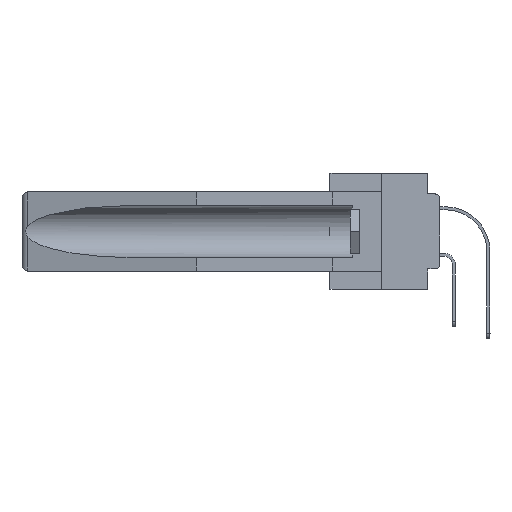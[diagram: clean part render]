
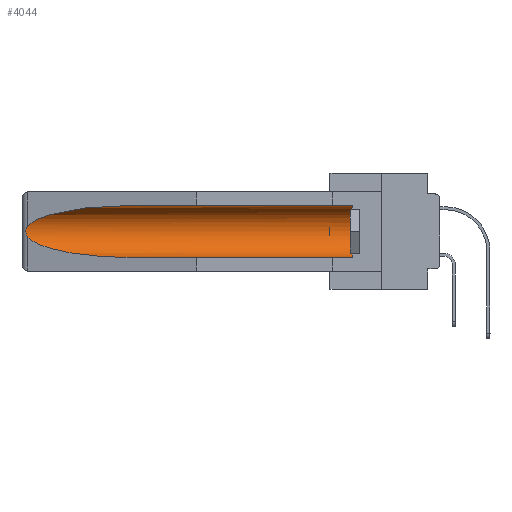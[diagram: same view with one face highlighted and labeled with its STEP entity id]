
A CAD part, left-side view. The second image highlights one B-rep face of the part: STEP entity #4044.
In plain terms, the highlighted cylindrical face has radius 2.857 mm (diameter 5.715 mm), a partial arc.
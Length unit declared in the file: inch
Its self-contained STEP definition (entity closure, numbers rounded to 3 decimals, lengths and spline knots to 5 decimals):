
#299 = CIRCLE ( 'NONE', #5809, 0.1125 ) ;
#533 = ORIENTED_EDGE ( 'NONE', *, *, #35859, .T. ) ;
#1902 = ORIENTED_EDGE ( 'NONE', *, *, #36746, .T. ) ;
#4044 = ADVANCED_FACE ( 'NONE', ( #23453 ), #39282, .F. ) ;
#4335 = CARTESIAN_POINT ( 'NONE',  ( 0.21114, 1.30732, -0.059 ) ) ;
#4344 = DIRECTION ( 'NONE',  ( 0., 1., 0. ) ) ;
#4730 = ORIENTED_EDGE ( 'NONE', *, *, #24050, .F. ) ;
#5407 = ORIENTED_EDGE ( 'NONE', *, *, #29648, .T. ) ;
#5632 = VERTEX_POINT ( 'NONE', #34740 ) ;
#5809 = AXIS2_PLACEMENT_3D ( 'NONE', #38741, #35045, #41558 ) ;
#7453 = CARTESIAN_POINT ( 'NONE',  ( 0.2675, 1.53308, -0.16763 ) ) ;
#7535 =( BOUNDED_CURVE ( )  B_SPLINE_CURVE ( 3, ( #8912, #19321, #12401, #36028 ),
 .UNSPECIFIED., .F., .F. ) 
 B_SPLINE_CURVE_WITH_KNOTS ( ( 4, 4 ),
 ( 0.1948, 1.5708 ),
 .UNSPECIFIED. ) 
 CURVE ( )  GEOMETRIC_REPRESENTATION_ITEM ( )  RATIONAL_B_SPLINE_CURVE ( ( 1., 0.848, 0.848, 1. ) ) 
 REPRESENTATION_ITEM ( '' )  );
#8299 = VECTOR ( 'NONE', #28967, 39.37008 ) ;
#8912 = CARTESIAN_POINT ( 'NONE',  ( 0.26537, 1.52718, -0.19328 ) ) ;
#8949 = CARTESIAN_POINT ( 'NONE',  ( 0.155, 1.07973, -0.284 ) ) ;
#11121 = CARTESIAN_POINT ( 'NONE',  ( 0.26597, 1.5296, -0.19026 ) ) ;
#12401 = CARTESIAN_POINT ( 'NONE',  ( 0.21114, 1.30732, -0.284 ) ) ;
#14147 = CARTESIAN_POINT ( 'NONE',  ( 0.2673, 1.5327, -0.16383 ) ) ;
#15965 = LINE ( 'NONE', #32635, #8299 ) ;
#16817 = CARTESIAN_POINT ( 'NONE',  ( 0.155, 0.126, -0.059 ) ) ;
#16933 = VERTEX_POINT ( 'NONE', #17651 ) ;
#17651 = CARTESIAN_POINT ( 'NONE',  ( 0.155, 1.07973, -0.059 ) ) ;
#17791 = AXIS2_PLACEMENT_3D ( 'NONE', #19331, #32550, #42531 ) ;
#18020 = CARTESIAN_POINT ( 'NONE',  ( 0.155, 0.126, -0.284 ) ) ;
#18270 =( BOUNDED_CURVE ( )  B_SPLINE_CURVE ( 3, ( #20996, #4335, #34221, #30986 ),
 .UNSPECIFIED., .F., .F. ) 
 B_SPLINE_CURVE_WITH_KNOTS ( ( 4, 4 ),
 ( 4.71239, 6.08839 ),
 .UNSPECIFIED. ) 
 CURVE ( )  GEOMETRIC_REPRESENTATION_ITEM ( )  RATIONAL_B_SPLINE_CURVE ( ( 1., 0.848, 0.848, 1. ) ) 
 REPRESENTATION_ITEM ( '' )  );
#19048 = EDGE_CURVE ( 'NONE', #34574, #16933, #34019, .T. ) ;
#19321 = CARTESIAN_POINT ( 'NONE',  ( 0.25451, 1.48313, -0.24835 ) ) ;
#19331 = CARTESIAN_POINT ( 'NONE',  ( 0.155, -0.30754, -0.1715 ) ) ;
#20863 = CARTESIAN_POINT ( 'NONE',  ( 0.2675, 1.53308, -0.17534 ) ) ;
#20996 = CARTESIAN_POINT ( 'NONE',  ( 0.155, 1.07973, -0.059 ) ) ;
#23453 = FACE_OUTER_BOUND ( 'NONE', #29745, .T. ) ;
#24050 = EDGE_CURVE ( 'NONE', #32086, #33594, #15965, .T. ) ;
#27362 = VECTOR ( 'NONE', #4344, 39.37008 ) ;
#27600 = CARTESIAN_POINT ( 'NONE',  ( 0.26655, 1.53094, -0.18657 ) ) ;
#28967 = DIRECTION ( 'NONE',  ( 0., 1., 0. ) ) ;
#29648 = EDGE_CURVE ( 'NONE', #16933, #35137, #18270, .T. ) ;
#29745 = EDGE_LOOP ( 'NONE', ( #5407, #38302, #533, #4730, #1902, #31126 ) ) ;
#30202 = CARTESIAN_POINT ( 'NONE',  ( 0.26654, 1.53092, -0.15636 ) ) ;
#30633 = CARTESIAN_POINT ( 'NONE',  ( 0.26537, 1.52718, -0.14972 ) ) ;
#30986 = CARTESIAN_POINT ( 'NONE',  ( 0.26537, 1.52718, -0.14972 ) ) ;
#31126 = ORIENTED_EDGE ( 'NONE', *, *, #19048, .T. ) ;
#32086 = VERTEX_POINT ( 'NONE', #18020 ) ;
#32550 = DIRECTION ( 'NONE',  ( 0., 1., 0. ) ) ;
#32635 = CARTESIAN_POINT ( 'NONE',  ( 0.155, -0.30754, -0.284 ) ) ;
#33454 = CARTESIAN_POINT ( 'NONE',  ( 0.26597, 1.52961, -0.15275 ) ) ;
#33594 = VERTEX_POINT ( 'NONE', #8949 ) ;
#34019 = LINE ( 'NONE', #37498, #27362 ) ;
#34088 = CARTESIAN_POINT ( 'NONE',  ( 0.2673, 1.53269, -0.17917 ) ) ;
#34221 = CARTESIAN_POINT ( 'NONE',  ( 0.25451, 1.48313, -0.09465 ) ) ;
#34574 = VERTEX_POINT ( 'NONE', #16817 ) ;
#34578 = B_SPLINE_CURVE_WITH_KNOTS ( 'NONE', 3,
 ( #30633, #33454, #30202, #14147, #7453, #20863, #34088, #27600, #11121, #37566 ),
 .UNSPECIFIED., .F., .F.,
 ( 4, 2, 2, 2, 4 ),
 ( 0., 0.00029, 0.00058, 0.00087, 0.00117 ),
 .UNSPECIFIED. ) ;
#34740 = CARTESIAN_POINT ( 'NONE',  ( 0.26537, 1.52718, -0.19328 ) ) ;
#35045 = DIRECTION ( 'NONE',  ( 0., -1., 0. ) ) ;
#35137 = VERTEX_POINT ( 'NONE', #37548 ) ;
#35859 = EDGE_CURVE ( 'NONE', #5632, #33594, #7535, .T. ) ;
#36028 = CARTESIAN_POINT ( 'NONE',  ( 0.155, 1.07973, -0.284 ) ) ;
#36746 = EDGE_CURVE ( 'NONE', #32086, #34574, #299, .T. ) ;
#37498 = CARTESIAN_POINT ( 'NONE',  ( 0.155, -0.30754, -0.059 ) ) ;
#37548 = CARTESIAN_POINT ( 'NONE',  ( 0.26537, 1.52718, -0.14972 ) ) ;
#37566 = CARTESIAN_POINT ( 'NONE',  ( 0.26537, 1.52718, -0.19328 ) ) ;
#37582 = EDGE_CURVE ( 'NONE', #35137, #5632, #34578, .T. ) ;
#38302 = ORIENTED_EDGE ( 'NONE', *, *, #37582, .T. ) ;
#38741 = CARTESIAN_POINT ( 'NONE',  ( 0.155, 0.126, -0.1715 ) ) ;
#39282 = CYLINDRICAL_SURFACE ( 'NONE', #17791, 0.1125 ) ;
#41558 = DIRECTION ( 'NONE',  ( 0., 0., 1. ) ) ;
#42531 = DIRECTION ( 'NONE',  ( 0., 0., 1. ) ) ;
